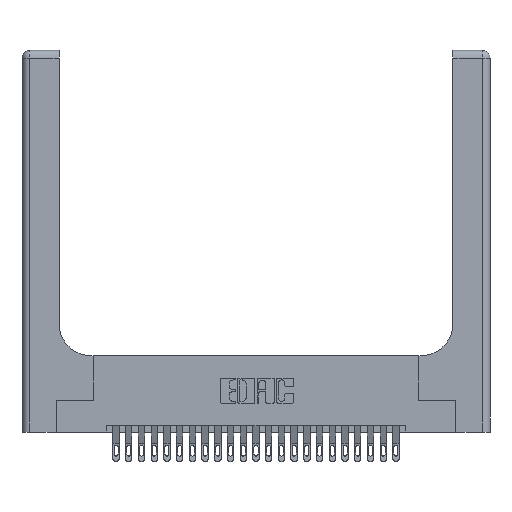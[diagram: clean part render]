
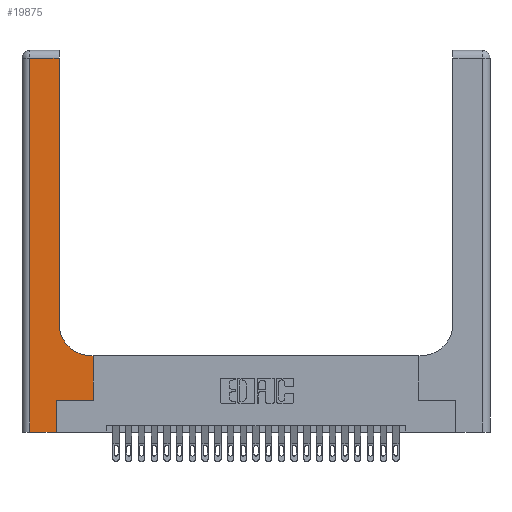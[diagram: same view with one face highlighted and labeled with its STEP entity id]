
A CAD part, top view. The second image highlights one B-rep face of the part: STEP entity #19875.
In plain terms, the highlighted planar face has unit normal (0, 0, 1).
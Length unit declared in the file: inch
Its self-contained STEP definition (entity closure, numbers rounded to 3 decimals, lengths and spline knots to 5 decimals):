
#213 = ORIENTED_EDGE ( 'NONE', *, *, #24670, .T. ) ;
#371 = DIRECTION ( 'NONE',  ( 0., 1., 0. ) ) ;
#589 = CARTESIAN_POINT ( 'NONE',  ( 0.5585, 0.6, 0.37 ) ) ;
#986 = DIRECTION ( 'NONE',  ( 0., 0., -1. ) ) ;
#1569 = ORIENTED_EDGE ( 'NONE', *, *, #5453, .T. ) ;
#2078 = DIRECTION ( 'NONE',  ( 0., 0., -1. ) ) ;
#3656 = CARTESIAN_POINT ( 'NONE',  ( 0., 3., 0.37 ) ) ;
#3863 = ORIENTED_EDGE ( 'NONE', *, *, #14754, .T. ) ;
#3883 = LINE ( 'NONE', #14353, #24781 ) ;
#4169 = CARTESIAN_POINT ( 'NONE',  ( 0.5415, 0.85, 0.37 ) ) ;
#4761 = VECTOR ( 'NONE', #16772, 39.37008 ) ;
#4945 = CARTESIAN_POINT ( 'NONE',  ( 0.2915, 3., 0.37 ) ) ;
#5139 = DIRECTION ( 'NONE',  ( -1., 0., 0. ) ) ;
#5143 = VECTOR ( 'NONE', #8663, 39.37008 ) ;
#5218 = CARTESIAN_POINT ( 'NONE',  ( 0.06, 0., 0.37 ) ) ;
#5230 = VERTEX_POINT ( 'NONE', #15164 ) ;
#5453 = EDGE_CURVE ( 'NONE', #8400, #14782, #6820, .T. ) ;
#6130 = CARTESIAN_POINT ( 'NONE',  ( 0.269, 0.25, 0.37 ) ) ;
#6399 = VECTOR ( 'NONE', #8760, 39.37008 ) ;
#6820 = LINE ( 'NONE', #20950, #17870 ) ;
#7582 = LINE ( 'NONE', #4945, #4761 ) ;
#7642 = VECTOR ( 'NONE', #15232, 39.37008 ) ;
#7653 = LINE ( 'NONE', #20760, #5143 ) ;
#7736 = VERTEX_POINT ( 'NONE', #9649 ) ;
#7894 = FACE_OUTER_BOUND ( 'NONE', #8775, .T. ) ;
#8400 = VERTEX_POINT ( 'NONE', #22185 ) ;
#8445 = LINE ( 'NONE', #24219, #25839 ) ;
#8663 = DIRECTION ( 'NONE',  ( 1., 0., 0. ) ) ;
#8760 = DIRECTION ( 'NONE',  ( 0., 1., 0. ) ) ;
#8775 = EDGE_LOOP ( 'NONE', ( #3863, #1569, #14618, #213, #13957, #18686, #25271, #12318, #19898 ) ) ;
#9649 = CARTESIAN_POINT ( 'NONE',  ( 0.5585, 0.25, 0.37 ) ) ;
#10298 = AXIS2_PLACEMENT_3D ( 'NONE', #4169, #2078, #12305 ) ;
#11189 = VERTEX_POINT ( 'NONE', #15726 ) ;
#11810 = LINE ( 'NONE', #14850, #6399 ) ;
#12051 = EDGE_CURVE ( 'NONE', #5230, #16409, #3883, .T. ) ;
#12147 = EDGE_CURVE ( 'NONE', #17180, #11189, #23477, .T. ) ;
#12305 = DIRECTION ( 'NONE',  ( 1., 0., 0. ) ) ;
#12318 = ORIENTED_EDGE ( 'NONE', *, *, #12147, .T. ) ;
#12811 = CARTESIAN_POINT ( 'NONE',  ( 0.06, 2.94, 0.37 ) ) ;
#13253 = CARTESIAN_POINT ( 'NONE',  ( 0.2915, 0.85, 0.37 ) ) ;
#13324 = EDGE_CURVE ( 'NONE', #7736, #17180, #11810, .T. ) ;
#13957 = ORIENTED_EDGE ( 'NONE', *, *, #12051, .T. ) ;
#14353 = CARTESIAN_POINT ( 'NONE',  ( 0.269, 0., 0.37 ) ) ;
#14618 = ORIENTED_EDGE ( 'NONE', *, *, #21573, .T. ) ;
#14754 = EDGE_CURVE ( 'NONE', #21835, #8400, #7582, .T. ) ;
#14782 = VERTEX_POINT ( 'NONE', #12811 ) ;
#14850 = CARTESIAN_POINT ( 'NONE',  ( 0.5585, 0.25, 0.37 ) ) ;
#15164 = CARTESIAN_POINT ( 'NONE',  ( 0.269, 0., 0.37 ) ) ;
#15232 = DIRECTION ( 'NONE',  ( -1., 0., 0. ) ) ;
#15726 = CARTESIAN_POINT ( 'NONE',  ( 0.5415, 0.6, 0.37 ) ) ;
#15888 = DIRECTION ( 'NONE',  ( 1., 0., 0. ) ) ;
#16409 = VERTEX_POINT ( 'NONE', #6130 ) ;
#16772 = DIRECTION ( 'NONE',  ( 0., 1., 0. ) ) ;
#17048 = VERTEX_POINT ( 'NONE', #5218 ) ;
#17100 = DIRECTION ( 'NONE',  ( -1., 0., 0. ) ) ;
#17180 = VERTEX_POINT ( 'NONE', #589 ) ;
#17870 = VECTOR ( 'NONE', #5139, 39.37008 ) ;
#18215 = EDGE_CURVE ( 'NONE', #11189, #21835, #19783, .T. ) ;
#18686 = ORIENTED_EDGE ( 'NONE', *, *, #20105, .T. ) ;
#18858 = PLANE ( 'NONE',  #21002 ) ;
#19783 = CIRCLE ( 'NONE', #10298, 0.25 ) ;
#19875 = ADVANCED_FACE ( 'NONE', ( #7894 ), #18858, .F. ) ;
#19898 = ORIENTED_EDGE ( 'NONE', *, *, #18215, .T. ) ;
#20105 = EDGE_CURVE ( 'NONE', #16409, #7736, #23408, .T. ) ;
#20760 = CARTESIAN_POINT ( 'NONE',  ( 0., 0., 0.37 ) ) ;
#20950 = CARTESIAN_POINT ( 'NONE',  ( 0., 2.94, 0.37 ) ) ;
#21002 = AXIS2_PLACEMENT_3D ( 'NONE', #3656, #986, #17100 ) ;
#21381 = CARTESIAN_POINT ( 'NONE',  ( 0.2915, 0.6, 0.37 ) ) ;
#21573 = EDGE_CURVE ( 'NONE', #14782, #17048, #8445, .T. ) ;
#21835 = VERTEX_POINT ( 'NONE', #13253 ) ;
#22185 = CARTESIAN_POINT ( 'NONE',  ( 0.2915, 2.94, 0.37 ) ) ;
#23082 = VECTOR ( 'NONE', #15888, 39.37008 ) ;
#23408 = LINE ( 'NONE', #24576, #23082 ) ;
#23477 = LINE ( 'NONE', #21381, #7642 ) ;
#24219 = CARTESIAN_POINT ( 'NONE',  ( 0.06, 3., 0.37 ) ) ;
#24298 = DIRECTION ( 'NONE',  ( 0., -1., 0. ) ) ;
#24576 = CARTESIAN_POINT ( 'NONE',  ( 0.269, 0.25, 0.37 ) ) ;
#24670 = EDGE_CURVE ( 'NONE', #17048, #5230, #7653, .T. ) ;
#24781 = VECTOR ( 'NONE', #371, 39.37008 ) ;
#25271 = ORIENTED_EDGE ( 'NONE', *, *, #13324, .T. ) ;
#25839 = VECTOR ( 'NONE', #24298, 39.37008 ) ;
